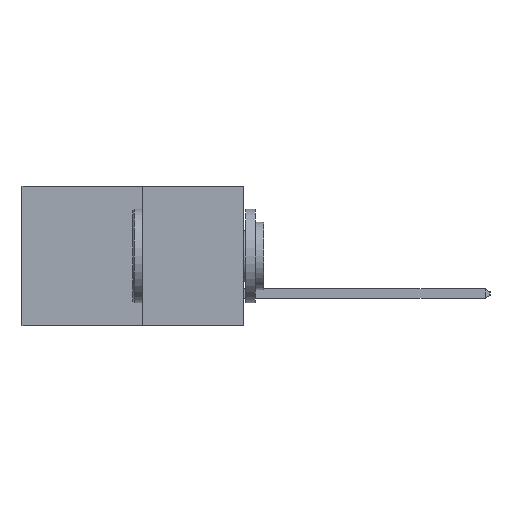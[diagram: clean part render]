
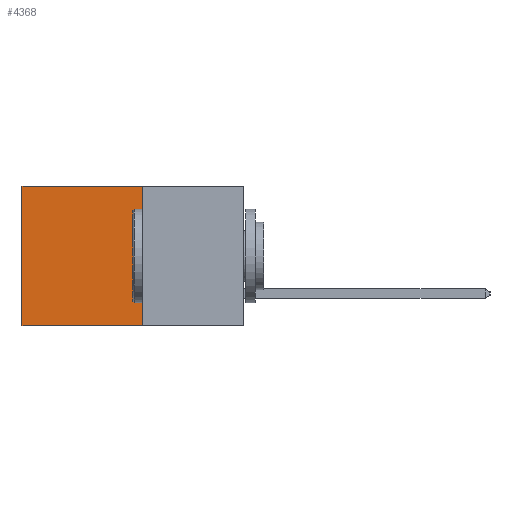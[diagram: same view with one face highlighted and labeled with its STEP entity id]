
A CAD part, left-side view. The second image highlights one B-rep face of the part: STEP entity #4368.
In plain terms, the highlighted planar face has unit normal (-1, 0, 0).
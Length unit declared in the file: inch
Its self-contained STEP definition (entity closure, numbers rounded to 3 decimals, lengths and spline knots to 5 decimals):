
#1528 = CARTESIAN_POINT ( 'NONE',  ( 0.277, 0.59, 0. ) ) ;
#1723 = PLANE ( 'NONE',  #9924 ) ;
#1733 = DIRECTION ( 'NONE',  ( 1., 0., 0. ) ) ;
#1891 = DIRECTION ( 'NONE',  ( 0., 1., 0. ) ) ;
#1925 = VECTOR ( 'NONE', #6577, 39.37008 ) ;
#1990 = CARTESIAN_POINT ( 'NONE',  ( 0.277, 0.27, 0. ) ) ;
#2221 = EDGE_CURVE ( 'NONE', #7175, #8326, #4819, .T. ) ;
#2582 = CARTESIAN_POINT ( 'NONE',  ( 0.277, 0.27, 0. ) ) ;
#3115 = EDGE_LOOP ( 'NONE', ( #10269, #3555, #8478, #4409 ) ) ;
#3203 = FACE_OUTER_BOUND ( 'NONE', #3115, .T. ) ;
#3555 = ORIENTED_EDGE ( 'NONE', *, *, #9778, .F. ) ;
#3579 = CARTESIAN_POINT ( 'NONE',  ( 0.277, 0.59, -0.37 ) ) ;
#3607 = DIRECTION ( 'NONE',  ( 0., 0., -1. ) ) ;
#3788 = EDGE_CURVE ( 'NONE', #5664, #11653, #4353, .T. ) ;
#4353 = LINE ( 'NONE', #5377, #1925 ) ;
#4368 = ADVANCED_FACE ( 'NONE', ( #3203 ), #1723, .F. ) ;
#4409 = ORIENTED_EDGE ( 'NONE', *, *, #7128, .T. ) ;
#4592 = VECTOR ( 'NONE', #7434, 39.37008 ) ;
#4819 = LINE ( 'NONE', #9018, #11704 ) ;
#5249 = DIRECTION ( 'NONE',  ( 0., 0., -1. ) ) ;
#5377 = CARTESIAN_POINT ( 'NONE',  ( 0.277, 0.27, -0.37 ) ) ;
#5529 = LINE ( 'NONE', #10925, #4592 ) ;
#5664 = VERTEX_POINT ( 'NONE', #2582 ) ;
#5962 = CARTESIAN_POINT ( 'NONE',  ( 0.277, 0.27, -0.37 ) ) ;
#5979 = CARTESIAN_POINT ( 'NONE',  ( 0.277, 0.27, -0.37 ) ) ;
#6577 = DIRECTION ( 'NONE',  ( 0., 0., -1. ) ) ;
#7128 = EDGE_CURVE ( 'NONE', #5664, #7175, #7178, .T. ) ;
#7175 = VERTEX_POINT ( 'NONE', #1528 ) ;
#7178 = LINE ( 'NONE', #1990, #9333 ) ;
#7434 = DIRECTION ( 'NONE',  ( 0., 1., 0. ) ) ;
#8326 = VERTEX_POINT ( 'NONE', #3579 ) ;
#8478 = ORIENTED_EDGE ( 'NONE', *, *, #3788, .F. ) ;
#9018 = CARTESIAN_POINT ( 'NONE',  ( 0.277, 0.59, -0.37 ) ) ;
#9333 = VECTOR ( 'NONE', #1891, 39.37008 ) ;
#9778 = EDGE_CURVE ( 'NONE', #11653, #8326, #5529, .T. ) ;
#9924 = AXIS2_PLACEMENT_3D ( 'NONE', #5962, #1733, #3607 ) ;
#10269 = ORIENTED_EDGE ( 'NONE', *, *, #2221, .T. ) ;
#10925 = CARTESIAN_POINT ( 'NONE',  ( 0.277, 0.27, -0.37 ) ) ;
#11653 = VERTEX_POINT ( 'NONE', #5979 ) ;
#11704 = VECTOR ( 'NONE', #5249, 39.37008 ) ;
